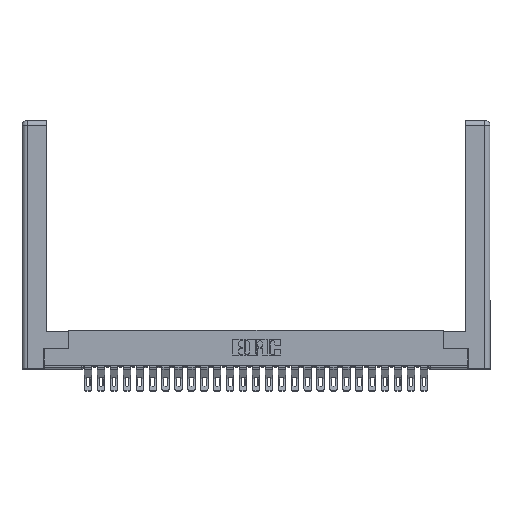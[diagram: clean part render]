
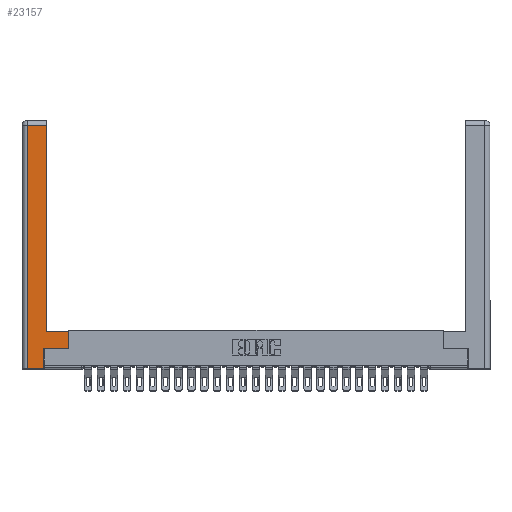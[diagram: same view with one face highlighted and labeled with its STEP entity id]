
A CAD part, top view. The second image highlights one B-rep face of the part: STEP entity #23157.
In plain terms, the highlighted planar face has unit normal (0, 0, 1).
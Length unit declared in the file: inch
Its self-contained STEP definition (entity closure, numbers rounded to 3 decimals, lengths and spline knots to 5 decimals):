
#56 = VECTOR ( 'NONE', #14507, 39.37008 ) ;
#77 = CARTESIAN_POINT ( 'NONE',  ( 0.295, 0.45, 0. ) ) ;
#366 = VERTEX_POINT ( 'NONE', #4645 ) ;
#491 = CARTESIAN_POINT ( 'NONE',  ( 0.565, 0.245, 0. ) ) ;
#1016 = DIRECTION ( 'NONE',  ( 0., 1., 0. ) ) ;
#1691 = LINE ( 'NONE', #77, #8024 ) ;
#1864 = VECTOR ( 'NONE', #21766, 39.37008 ) ;
#2029 = VERTEX_POINT ( 'NONE', #4539 ) ;
#3071 = CARTESIAN_POINT ( 'NONE',  ( 0., 0., 0. ) ) ;
#3905 = ORIENTED_EDGE ( 'NONE', *, *, #27807, .T. ) ;
#4120 = VERTEX_POINT ( 'NONE', #18903 ) ;
#4165 = DIRECTION ( 'NONE',  ( 0., 1., 0. ) ) ;
#4271 = VERTEX_POINT ( 'NONE', #24145 ) ;
#4539 = CARTESIAN_POINT ( 'NONE',  ( 0.295, 2.94, 0. ) ) ;
#4645 = CARTESIAN_POINT ( 'NONE',  ( 0.265, 0.245, 0. ) ) ;
#4736 = DIRECTION ( 'NONE',  ( 0., -1., 0. ) ) ;
#5024 = VERTEX_POINT ( 'NONE', #13876 ) ;
#6761 = LINE ( 'NONE', #23455, #56 ) ;
#6944 = VECTOR ( 'NONE', #11620, 39.37008 ) ;
#7960 = ORIENTED_EDGE ( 'NONE', *, *, #24087, .T. ) ;
#8024 = VECTOR ( 'NONE', #24921, 39.37008 ) ;
#8331 = ORIENTED_EDGE ( 'NONE', *, *, #15804, .T. ) ;
#9047 = DIRECTION ( 'NONE',  ( 1., 0., 0. ) ) ;
#9067 = LINE ( 'NONE', #491, #6944 ) ;
#9263 = CARTESIAN_POINT ( 'NONE',  ( 0.0615, 0., 0. ) ) ;
#9285 = LINE ( 'NONE', #28732, #1864 ) ;
#9679 = CARTESIAN_POINT ( 'NONE',  ( 0.265, 0., 0. ) ) ;
#10346 = LINE ( 'NONE', #13180, #17693 ) ;
#10662 = LINE ( 'NONE', #28011, #27832 ) ;
#10852 = ORIENTED_EDGE ( 'NONE', *, *, #16193, .T. ) ;
#10979 = EDGE_CURVE ( 'NONE', #2029, #4271, #9285, .T. ) ;
#11283 = ORIENTED_EDGE ( 'NONE', *, *, #10979, .T. ) ;
#11620 = DIRECTION ( 'NONE',  ( 1., 0., 0. ) ) ;
#11926 = VERTEX_POINT ( 'NONE', #24246 ) ;
#12142 = AXIS2_PLACEMENT_3D ( 'NONE', #3071, #16705, #20920 ) ;
#13180 = CARTESIAN_POINT ( 'NONE',  ( 0.295, 3., 0. ) ) ;
#13631 = VECTOR ( 'NONE', #4736, 39.37008 ) ;
#13876 = CARTESIAN_POINT ( 'NONE',  ( 0.565, 0.245, 0. ) ) ;
#14373 = EDGE_CURVE ( 'NONE', #4120, #20802, #17895, .T. ) ;
#14507 = DIRECTION ( 'NONE',  ( 0., 1., 0. ) ) ;
#15777 = CARTESIAN_POINT ( 'NONE',  ( 0.265, 0., 0. ) ) ;
#15804 = EDGE_CURVE ( 'NONE', #4271, #4120, #19551, .T. ) ;
#16193 = EDGE_CURVE ( 'NONE', #366, #5024, #9067, .T. ) ;
#16364 = CARTESIAN_POINT ( 'NONE',  ( 0.295, 0.45, 0. ) ) ;
#16705 = DIRECTION ( 'NONE',  ( 0., 0., -1. ) ) ;
#17516 = FACE_OUTER_BOUND ( 'NONE', #27621, .T. ) ;
#17693 = VECTOR ( 'NONE', #4165, 39.37008 ) ;
#17895 = LINE ( 'NONE', #15777, #22437 ) ;
#17940 = EDGE_CURVE ( 'NONE', #26680, #2029, #10346, .T. ) ;
#18553 = PLANE ( 'NONE',  #12142 ) ;
#18903 = CARTESIAN_POINT ( 'NONE',  ( 0.0615, 0., 0. ) ) ;
#19551 = LINE ( 'NONE', #9263, #13631 ) ;
#20449 = ORIENTED_EDGE ( 'NONE', *, *, #14373, .T. ) ;
#20802 = VERTEX_POINT ( 'NONE', #9679 ) ;
#20920 = DIRECTION ( 'NONE',  ( -1., 0., 0. ) ) ;
#21766 = DIRECTION ( 'NONE',  ( -1., 0., 0. ) ) ;
#22437 = VECTOR ( 'NONE', #9047, 39.37008 ) ;
#23038 = ORIENTED_EDGE ( 'NONE', *, *, #17940, .T. ) ;
#23157 = ADVANCED_FACE ( 'NONE', ( #17516 ), #18553, .F. ) ;
#23455 = CARTESIAN_POINT ( 'NONE',  ( 0.265, 0.245, 0. ) ) ;
#24087 = EDGE_CURVE ( 'NONE', #11926, #26680, #1691, .T. ) ;
#24145 = CARTESIAN_POINT ( 'NONE',  ( 0.0615, 2.94, 0. ) ) ;
#24246 = CARTESIAN_POINT ( 'NONE',  ( 0.565, 0.45, 0. ) ) ;
#24921 = DIRECTION ( 'NONE',  ( -1., 0., 0. ) ) ;
#25748 = ORIENTED_EDGE ( 'NONE', *, *, #28620, .T. ) ;
#26680 = VERTEX_POINT ( 'NONE', #16364 ) ;
#27621 = EDGE_LOOP ( 'NONE', ( #23038, #11283, #8331, #20449, #25748, #10852, #3905, #7960 ) ) ;
#27807 = EDGE_CURVE ( 'NONE', #5024, #11926, #10662, .T. ) ;
#27832 = VECTOR ( 'NONE', #1016, 39.37008 ) ;
#28011 = CARTESIAN_POINT ( 'NONE',  ( 0.565, 0.45, 0. ) ) ;
#28620 = EDGE_CURVE ( 'NONE', #20802, #366, #6761, .T. ) ;
#28732 = CARTESIAN_POINT ( 'NONE',  ( 0.0615, 2.94, 0. ) ) ;
